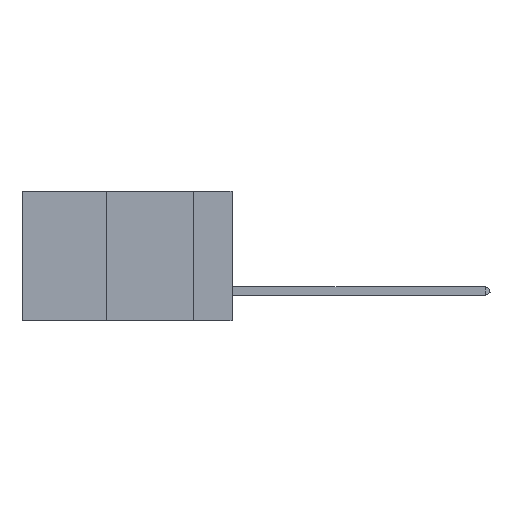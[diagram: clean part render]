
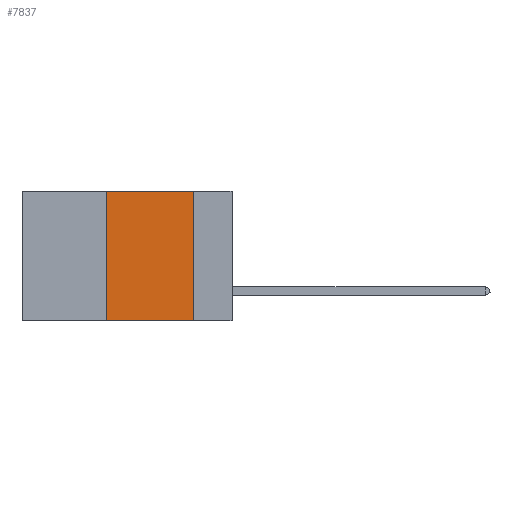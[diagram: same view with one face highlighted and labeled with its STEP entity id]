
A CAD part, left-side view. The second image highlights one B-rep face of the part: STEP entity #7837.
In plain terms, the highlighted planar face has unit normal (-1, 0, 0).
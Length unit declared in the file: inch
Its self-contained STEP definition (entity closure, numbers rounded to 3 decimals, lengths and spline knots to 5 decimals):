
#870 = DIRECTION ( 'NONE',  ( 0., 0., -1. ) ) ;
#1163 = EDGE_CURVE ( 'NONE', #8562, #10304, #3424, .T. ) ;
#2296 = DIRECTION ( 'NONE',  ( 1., 0., 0. ) ) ;
#2350 = LINE ( 'NONE', #7953, #11732 ) ;
#2699 = ORIENTED_EDGE ( 'NONE', *, *, #1163, .F. ) ;
#2803 = EDGE_CURVE ( 'NONE', #6921, #7932, #9917, .T. ) ;
#3145 = FACE_OUTER_BOUND ( 'NONE', #7795, .T. ) ;
#3167 = ORIENTED_EDGE ( 'NONE', *, *, #6092, .T. ) ;
#3424 = LINE ( 'NONE', #7209, #8517 ) ;
#3596 = DIRECTION ( 'NONE',  ( 0., 0., 1. ) ) ;
#4632 = CARTESIAN_POINT ( 'NONE',  ( 0., 0.11, 0. ) ) ;
#4781 = CARTESIAN_POINT ( 'NONE',  ( 0., 0.11, 0. ) ) ;
#4812 = ORIENTED_EDGE ( 'NONE', *, *, #2803, .F. ) ;
#4914 = CARTESIAN_POINT ( 'NONE',  ( 0., 0.6, 0. ) ) ;
#5050 = EDGE_CURVE ( 'NONE', #10304, #6921, #2350, .T. ) ;
#5796 = CARTESIAN_POINT ( 'NONE',  ( 0., 0.36, -0.37 ) ) ;
#6092 = EDGE_CURVE ( 'NONE', #8562, #7932, #6690, .T. ) ;
#6237 = CARTESIAN_POINT ( 'NONE',  ( 0., 0.11, -0.37 ) ) ;
#6690 = LINE ( 'NONE', #7113, #9283 ) ;
#6921 = VERTEX_POINT ( 'NONE', #4781 ) ;
#7034 = VECTOR ( 'NONE', #870, 39.37008 ) ;
#7113 = CARTESIAN_POINT ( 'NONE',  ( 0., 0.6, -0.37 ) ) ;
#7209 = CARTESIAN_POINT ( 'NONE',  ( 0., 0.36, 0. ) ) ;
#7715 = PLANE ( 'NONE',  #7791 ) ;
#7791 = AXIS2_PLACEMENT_3D ( 'NONE', #4914, #2296, #8631 ) ;
#7795 = EDGE_LOOP ( 'NONE', ( #4812, #10044, #2699, #3167 ) ) ;
#7836 = DIRECTION ( 'NONE',  ( 0., -1., 0. ) ) ;
#7837 = ADVANCED_FACE ( 'NONE', ( #3145 ), #7715, .F. ) ;
#7932 = VERTEX_POINT ( 'NONE', #6237 ) ;
#7953 = CARTESIAN_POINT ( 'NONE',  ( 0., 0.6, 0. ) ) ;
#8411 = CARTESIAN_POINT ( 'NONE',  ( 0., 0.36, 0. ) ) ;
#8517 = VECTOR ( 'NONE', #3596, 39.37008 ) ;
#8562 = VERTEX_POINT ( 'NONE', #5796 ) ;
#8631 = DIRECTION ( 'NONE',  ( 0., 0., -1. ) ) ;
#8679 = DIRECTION ( 'NONE',  ( 0., -1., 0. ) ) ;
#9283 = VECTOR ( 'NONE', #7836, 39.37008 ) ;
#9917 = LINE ( 'NONE', #4632, #7034 ) ;
#10044 = ORIENTED_EDGE ( 'NONE', *, *, #5050, .F. ) ;
#10304 = VERTEX_POINT ( 'NONE', #8411 ) ;
#11732 = VECTOR ( 'NONE', #8679, 39.37008 ) ;
